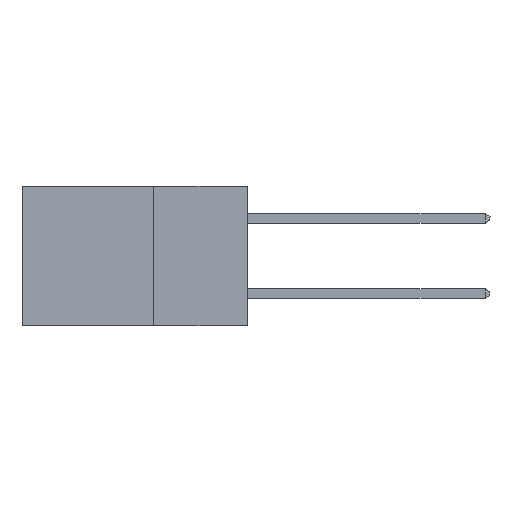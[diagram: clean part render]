
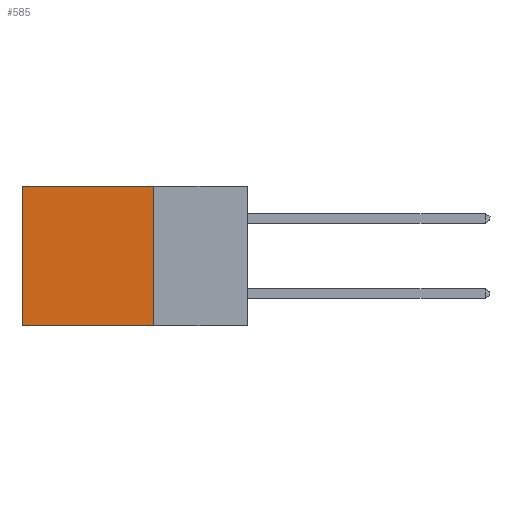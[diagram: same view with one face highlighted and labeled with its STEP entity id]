
A CAD part, left-side view. The second image highlights one B-rep face of the part: STEP entity #585.
In plain terms, the highlighted planar face has unit normal (-1, 0, 0).
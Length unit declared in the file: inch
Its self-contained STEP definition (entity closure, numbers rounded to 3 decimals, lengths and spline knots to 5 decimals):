
#215 = PLANE ( 'NONE',  #928 ) ;
#403 = CARTESIAN_POINT ( 'NONE',  ( 0.2615, 0.25, -0.37 ) ) ;
#431 = VERTEX_POINT ( 'NONE', #7946 ) ;
#568 = DIRECTION ( 'NONE',  ( 0., 0., -1. ) ) ;
#585 = ADVANCED_FACE ( 'NONE', ( #6248 ), #215, .F. ) ;
#928 = AXIS2_PLACEMENT_3D ( 'NONE', #7193, #5486, #2747 ) ;
#1045 = VERTEX_POINT ( 'NONE', #10247 ) ;
#1391 = LINE ( 'NONE', #403, #8236 ) ;
#1596 = CARTESIAN_POINT ( 'NONE',  ( 0.2615, 0.25, 0. ) ) ;
#1941 = EDGE_CURVE ( 'NONE', #1045, #4935, #1391, .T. ) ;
#2062 = EDGE_CURVE ( 'NONE', #431, #8068, #10274, .T. ) ;
#2377 = LINE ( 'NONE', #1596, #3136 ) ;
#2747 = DIRECTION ( 'NONE',  ( 0., 0., -1. ) ) ;
#3136 = VECTOR ( 'NONE', #5870, 39.37008 ) ;
#3158 = VECTOR ( 'NONE', #4060, 39.37008 ) ;
#3581 = CARTESIAN_POINT ( 'NONE',  ( 0.2615, 0.6, -0.37 ) ) ;
#3999 = CARTESIAN_POINT ( 'NONE',  ( 0.2615, 0.25, -0.37 ) ) ;
#4060 = DIRECTION ( 'NONE',  ( 0., 1., 0. ) ) ;
#4176 = EDGE_CURVE ( 'NONE', #1045, #431, #2377, .T. ) ;
#4514 = EDGE_LOOP ( 'NONE', ( #10537, #11198, #7060, #4893 ) ) ;
#4893 = ORIENTED_EDGE ( 'NONE', *, *, #4176, .T. ) ;
#4935 = VERTEX_POINT ( 'NONE', #3999 ) ;
#5486 = DIRECTION ( 'NONE',  ( 1., 0., 0. ) ) ;
#5537 = EDGE_CURVE ( 'NONE', #4935, #8068, #5889, .T. ) ;
#5870 = DIRECTION ( 'NONE',  ( 0., 1., 0. ) ) ;
#5889 = LINE ( 'NONE', #7538, #3158 ) ;
#6248 = FACE_OUTER_BOUND ( 'NONE', #4514, .T. ) ;
#6255 = VECTOR ( 'NONE', #568, 39.37008 ) ;
#7060 = ORIENTED_EDGE ( 'NONE', *, *, #1941, .F. ) ;
#7193 = CARTESIAN_POINT ( 'NONE',  ( 0.2615, 0.25, -0.37 ) ) ;
#7538 = CARTESIAN_POINT ( 'NONE',  ( 0.2615, 0.25, -0.37 ) ) ;
#7540 = CARTESIAN_POINT ( 'NONE',  ( 0.2615, 0.6, -0.37 ) ) ;
#7946 = CARTESIAN_POINT ( 'NONE',  ( 0.2615, 0.6, 0. ) ) ;
#8068 = VERTEX_POINT ( 'NONE', #3581 ) ;
#8236 = VECTOR ( 'NONE', #10743, 39.37008 ) ;
#10247 = CARTESIAN_POINT ( 'NONE',  ( 0.2615, 0.25, 0. ) ) ;
#10274 = LINE ( 'NONE', #7540, #6255 ) ;
#10537 = ORIENTED_EDGE ( 'NONE', *, *, #2062, .T. ) ;
#10743 = DIRECTION ( 'NONE',  ( 0., 0., -1. ) ) ;
#11198 = ORIENTED_EDGE ( 'NONE', *, *, #5537, .F. ) ;
